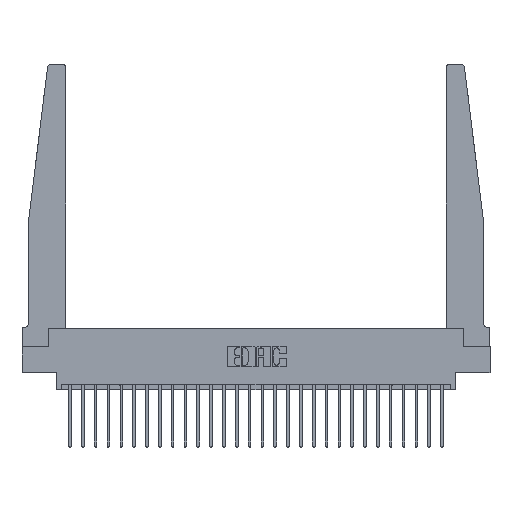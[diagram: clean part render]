
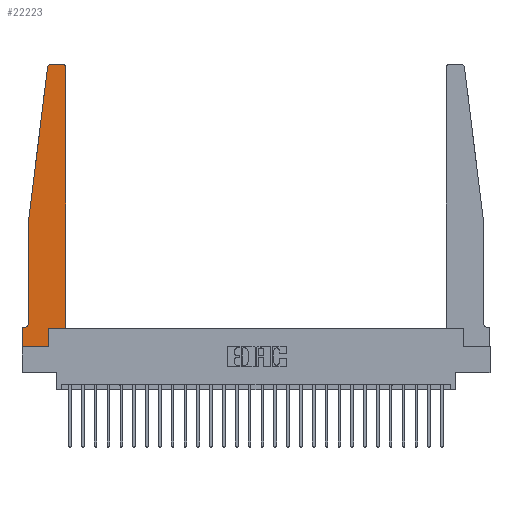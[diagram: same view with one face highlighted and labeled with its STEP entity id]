
A CAD part, top view. The second image highlights one B-rep face of the part: STEP entity #22223.
In plain terms, the highlighted planar face has unit normal (0, 0, 1).
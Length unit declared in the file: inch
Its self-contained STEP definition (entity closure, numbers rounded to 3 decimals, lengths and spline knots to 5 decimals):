
#264 = ORIENTED_EDGE ( 'NONE', *, *, #23495, .T. ) ;
#643 = DIRECTION ( 'NONE',  ( 0., -1., 0. ) ) ;
#877 = EDGE_LOOP ( 'NONE', ( #264, #22319, #9364, #2571, #22508, #10941, #25907, #14437, #1449, #2940, #3910, #24144 ) ) ;
#971 = VERTEX_POINT ( 'NONE', #11088 ) ;
#1042 = DIRECTION ( 'NONE',  ( 0., 1., 0. ) ) ;
#1156 = CIRCLE ( 'NONE', #10102, 0.03 ) ;
#1449 = ORIENTED_EDGE ( 'NONE', *, *, #23974, .T. ) ;
#1538 = LINE ( 'NONE', #17916, #26459 ) ;
#1721 = LINE ( 'NONE', #26312, #16331 ) ;
#1775 = CARTESIAN_POINT ( 'NONE',  ( 0.425, 0.18, 0.37 ) ) ;
#2022 = DIRECTION ( 'NONE',  ( -0.122, -0.992, 0. ) ) ;
#2136 = CARTESIAN_POINT ( 'NONE',  ( 0.065, 0.2375, 0.37 ) ) ;
#2154 = CARTESIAN_POINT ( 'NONE',  ( 0.065, 1.25, 0.37 ) ) ;
#2545 = CARTESIAN_POINT ( 'NONE',  ( 0.015, 0.1875, 0.37 ) ) ;
#2571 = ORIENTED_EDGE ( 'NONE', *, *, #3960, .T. ) ;
#2940 = ORIENTED_EDGE ( 'NONE', *, *, #14554, .T. ) ;
#3436 = DIRECTION ( 'NONE',  ( -1., 0., 0. ) ) ;
#3910 = ORIENTED_EDGE ( 'NONE', *, *, #5533, .T. ) ;
#3960 = EDGE_CURVE ( 'NONE', #25469, #19130, #1721, .T. ) ;
#4346 = EDGE_CURVE ( 'NONE', #12191, #13477, #18017, .T. ) ;
#4662 = VECTOR ( 'NONE', #19505, 39.37008 ) ;
#4856 = CARTESIAN_POINT ( 'NONE',  ( 0.065, 0.1875, 0.37 ) ) ;
#5178 = DIRECTION ( 'NONE',  ( 0., 0., 1. ) ) ;
#5533 = EDGE_CURVE ( 'NONE', #971, #14514, #23893, .T. ) ;
#6958 = VECTOR ( 'NONE', #1042, 39.37008 ) ;
#7271 = CARTESIAN_POINT ( 'NONE',  ( 0.2605, 0.18, 0.37 ) ) ;
#7295 = DIRECTION ( 'NONE',  ( 1., 0., 0. ) ) ;
#7693 = LINE ( 'NONE', #15935, #10526 ) ;
#8546 = DIRECTION ( 'NONE',  ( 0., 0., 1. ) ) ;
#9364 = ORIENTED_EDGE ( 'NONE', *, *, #24312, .T. ) ;
#9565 = DIRECTION ( 'NONE',  ( 1., 0., 0. ) ) ;
#9659 = EDGE_CURVE ( 'NONE', #10887, #26436, #25579, .T. ) ;
#9916 = DIRECTION ( 'NONE',  ( 1., 0., 0. ) ) ;
#10102 = AXIS2_PLACEMENT_3D ( 'NONE', #18934, #8546, #12769 ) ;
#10526 = VECTOR ( 'NONE', #3436, 39.37008 ) ;
#10562 = VECTOR ( 'NONE', #25170, 39.37008 ) ;
#10698 = CARTESIAN_POINT ( 'NONE',  ( 0., 0., 0.37 ) ) ;
#10868 = VERTEX_POINT ( 'NONE', #12625 ) ;
#10887 = VERTEX_POINT ( 'NONE', #2545 ) ;
#10897 = CARTESIAN_POINT ( 'NONE',  ( 0., 0., 0.37 ) ) ;
#10941 = ORIENTED_EDGE ( 'NONE', *, *, #9659, .T. ) ;
#11080 = EDGE_CURVE ( 'NONE', #19130, #10887, #22167, .T. ) ;
#11088 = CARTESIAN_POINT ( 'NONE',  ( 0.425, 0.18, 0.37 ) ) ;
#11624 = FACE_OUTER_BOUND ( 'NONE', #877, .T. ) ;
#11762 = CARTESIAN_POINT ( 'NONE',  ( 0.015, 0.2375, 0.37 ) ) ;
#12191 = VERTEX_POINT ( 'NONE', #25013 ) ;
#12625 = CARTESIAN_POINT ( 'NONE',  ( 0.2605, 0., 0.37 ) ) ;
#12740 = AXIS2_PLACEMENT_3D ( 'NONE', #11762, #26166, #18072 ) ;
#12756 = VECTOR ( 'NONE', #2022, 39.37008 ) ;
#12769 = DIRECTION ( 'NONE',  ( 1., 0., 0. ) ) ;
#12992 = VECTOR ( 'NONE', #14348, 39.37008 ) ;
#13057 = CARTESIAN_POINT ( 'NONE',  ( 0., 0., 0.37 ) ) ;
#13477 = VERTEX_POINT ( 'NONE', #18290 ) ;
#13754 = DIRECTION ( 'NONE',  ( 0., 1., 0. ) ) ;
#14348 = DIRECTION ( 'NONE',  ( 0., -1., 0. ) ) ;
#14437 = ORIENTED_EDGE ( 'NONE', *, *, #26054, .T. ) ;
#14514 = VERTEX_POINT ( 'NONE', #16005 ) ;
#14554 = EDGE_CURVE ( 'NONE', #23734, #971, #22346, .T. ) ;
#15632 = EDGE_CURVE ( 'NONE', #26436, #19691, #20939, .T. ) ;
#15935 = CARTESIAN_POINT ( 'NONE',  ( 0.25, 2.75, 0.37 ) ) ;
#16005 = CARTESIAN_POINT ( 'NONE',  ( 0.425, 2.72, 0.37 ) ) ;
#16331 = VECTOR ( 'NONE', #643, 39.37008 ) ;
#17293 = CARTESIAN_POINT ( 'NONE',  ( 0.425, 0.18, 0.37 ) ) ;
#17916 = CARTESIAN_POINT ( 'NONE',  ( 0.2605, 0.18, 0.37 ) ) ;
#18017 = CIRCLE ( 'NONE', #25766, 0.03 ) ;
#18072 = DIRECTION ( 'NONE',  ( -1., 0., 0. ) ) ;
#18290 = CARTESIAN_POINT ( 'NONE',  ( 0.24675, 2.72367, 0.37 ) ) ;
#18399 = LINE ( 'NONE', #2154, #12756 ) ;
#18934 = CARTESIAN_POINT ( 'NONE',  ( 0.395, 2.72, 0.37 ) ) ;
#19130 = VERTEX_POINT ( 'NONE', #2136 ) ;
#19504 = AXIS2_PLACEMENT_3D ( 'NONE', #19711, #5178, #7295 ) ;
#19505 = DIRECTION ( 'NONE',  ( -1., 0., 0. ) ) ;
#19691 = VERTEX_POINT ( 'NONE', #10897 ) ;
#19711 = CARTESIAN_POINT ( 'NONE',  ( 0., 0.1875, 0.37 ) ) ;
#19841 = PLANE ( 'NONE',  #19504 ) ;
#20939 = LINE ( 'NONE', #10698, #12992 ) ;
#22125 = CARTESIAN_POINT ( 'NONE',  ( 0.27653, 2.72, 0.37 ) ) ;
#22167 = CIRCLE ( 'NONE', #12740, 0.05 ) ;
#22223 = ADVANCED_FACE ( 'NONE', ( #11624 ), #19841, .T. ) ;
#22319 = ORIENTED_EDGE ( 'NONE', *, *, #4346, .T. ) ;
#22346 = LINE ( 'NONE', #1775, #25423 ) ;
#22508 = ORIENTED_EDGE ( 'NONE', *, *, #11080, .T. ) ;
#22663 = CARTESIAN_POINT ( 'NONE',  ( 0.065, 1.25, 0.37 ) ) ;
#23495 = EDGE_CURVE ( 'NONE', #23530, #12191, #7693, .T. ) ;
#23530 = VERTEX_POINT ( 'NONE', #24720 ) ;
#23734 = VERTEX_POINT ( 'NONE', #7271 ) ;
#23893 = LINE ( 'NONE', #17293, #6958 ) ;
#23974 = EDGE_CURVE ( 'NONE', #10868, #23734, #1538, .T. ) ;
#24022 = DIRECTION ( 'NONE',  ( 0., 0., 1. ) ) ;
#24144 = ORIENTED_EDGE ( 'NONE', *, *, #24494, .T. ) ;
#24312 = EDGE_CURVE ( 'NONE', #13477, #25469, #18399, .T. ) ;
#24494 = EDGE_CURVE ( 'NONE', #14514, #23530, #1156, .T. ) ;
#24720 = CARTESIAN_POINT ( 'NONE',  ( 0.395, 2.75, 0.37 ) ) ;
#25013 = CARTESIAN_POINT ( 'NONE',  ( 0.27653, 2.75, 0.37 ) ) ;
#25170 = DIRECTION ( 'NONE',  ( 1., 0., 0. ) ) ;
#25423 = VECTOR ( 'NONE', #9916, 39.37008 ) ;
#25469 = VERTEX_POINT ( 'NONE', #22663 ) ;
#25579 = LINE ( 'NONE', #4856, #4662 ) ;
#25632 = CARTESIAN_POINT ( 'NONE',  ( 0., 0.1875, 0.37 ) ) ;
#25689 = LINE ( 'NONE', #13057, #10562 ) ;
#25766 = AXIS2_PLACEMENT_3D ( 'NONE', #22125, #24022, #9565 ) ;
#25907 = ORIENTED_EDGE ( 'NONE', *, *, #15632, .T. ) ;
#26054 = EDGE_CURVE ( 'NONE', #19691, #10868, #25689, .T. ) ;
#26166 = DIRECTION ( 'NONE',  ( 0., 0., -1. ) ) ;
#26312 = CARTESIAN_POINT ( 'NONE',  ( 0.065, 1.25, 0.37 ) ) ;
#26436 = VERTEX_POINT ( 'NONE', #25632 ) ;
#26459 = VECTOR ( 'NONE', #13754, 39.37008 ) ;
